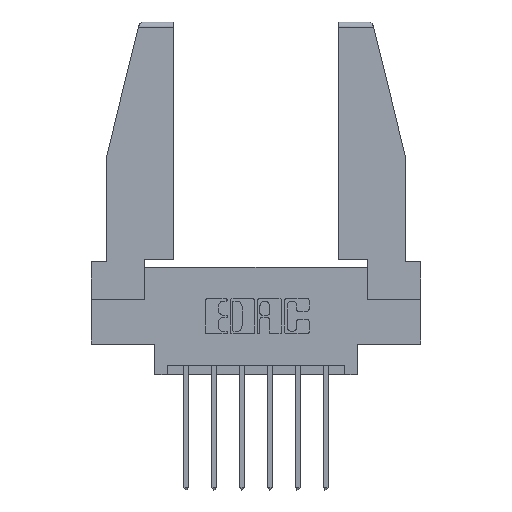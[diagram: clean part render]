
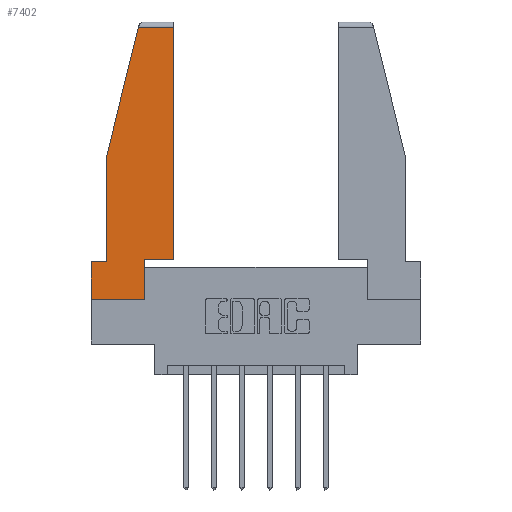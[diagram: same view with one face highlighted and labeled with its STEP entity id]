
A CAD part, top view. The second image highlights one B-rep face of the part: STEP entity #7402.
In plain terms, the highlighted planar face has unit normal (0, 0, 1).
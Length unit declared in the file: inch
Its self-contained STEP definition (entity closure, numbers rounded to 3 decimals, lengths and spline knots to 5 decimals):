
#170 = CARTESIAN_POINT ( 'NONE',  ( 0.297, 0.223, 0. ) ) ;
#223 = CARTESIAN_POINT ( 'NONE',  ( 0., 0.21, 0. ) ) ;
#345 = LINE ( 'NONE', #7909, #9709 ) ;
#404 = LINE ( 'NONE', #3564, #4568 ) ;
#1439 = EDGE_CURVE ( 'NONE', #1701, #2005, #3739, .T. ) ;
#1701 = VERTEX_POINT ( 'NONE', #3784 ) ;
#1802 = EDGE_CURVE ( 'NONE', #5195, #8325, #3585, .T. ) ;
#2005 = VERTEX_POINT ( 'NONE', #3179 ) ;
#2023 = DIRECTION ( 'NONE',  ( 1., 0., 0. ) ) ;
#2244 = CARTESIAN_POINT ( 'NONE',  ( 0., 0.21, 0. ) ) ;
#2677 = ORIENTED_EDGE ( 'NONE', *, *, #5609, .T. ) ;
#2774 = DIRECTION ( 'NONE',  ( 0., 1., 0. ) ) ;
#2810 = EDGE_CURVE ( 'NONE', #11155, #5195, #404, .T. ) ;
#3001 = ORIENTED_EDGE ( 'NONE', *, *, #6507, .T. ) ;
#3090 = ORIENTED_EDGE ( 'NONE', *, *, #7437, .T. ) ;
#3179 = CARTESIAN_POINT ( 'NONE',  ( 0.2636, 1.52, 0. ) ) ;
#3564 = CARTESIAN_POINT ( 'NONE',  ( 0.297, 0., 0. ) ) ;
#3585 = LINE ( 'NONE', #170, #5613 ) ;
#3739 = LINE ( 'NONE', #4511, #7657 ) ;
#3743 = DIRECTION ( 'NONE',  ( 1., 0., 0. ) ) ;
#3766 = CARTESIAN_POINT ( 'NONE',  ( 0., 0., 0. ) ) ;
#3771 = ORIENTED_EDGE ( 'NONE', *, *, #2810, .T. ) ;
#3784 = CARTESIAN_POINT ( 'NONE',  ( 0.461, 1.52, 0. ) ) ;
#4359 = EDGE_CURVE ( 'NONE', #9362, #11155, #7154, .T. ) ;
#4459 = CARTESIAN_POINT ( 'NONE',  ( 0.461, 0.223, 0. ) ) ;
#4460 = ORIENTED_EDGE ( 'NONE', *, *, #1802, .T. ) ;
#4511 = CARTESIAN_POINT ( 'NONE',  ( 0., 1.52, 0. ) ) ;
#4568 = VECTOR ( 'NONE', #5433, 39.37008 ) ;
#4641 = DIRECTION ( 'NONE',  ( -1., 0., 0. ) ) ;
#5174 = CARTESIAN_POINT ( 'NONE',  ( 0.297, 0.223, 0. ) ) ;
#5195 = VERTEX_POINT ( 'NONE', #5174 ) ;
#5255 = CARTESIAN_POINT ( 'NONE',  ( 0.297, 0., 0. ) ) ;
#5374 = DIRECTION ( 'NONE',  ( 0., -1., 0. ) ) ;
#5433 = DIRECTION ( 'NONE',  ( 0., 1., 0. ) ) ;
#5609 = EDGE_CURVE ( 'NONE', #8325, #1701, #7574, .T. ) ;
#5613 = VECTOR ( 'NONE', #3743, 39.37008 ) ;
#5628 = VERTEX_POINT ( 'NONE', #11048 ) ;
#5630 = CARTESIAN_POINT ( 'NONE',  ( 0., 0.21, 0. ) ) ;
#5664 = AXIS2_PLACEMENT_3D ( 'NONE', #3766, #7307, #10235 ) ;
#6057 = EDGE_CURVE ( 'NONE', #11297, #5628, #10888, .T. ) ;
#6272 = CARTESIAN_POINT ( 'NONE',  ( 0., 0., 0. ) ) ;
#6496 = VECTOR ( 'NONE', #8395, 39.37008 ) ;
#6507 = EDGE_CURVE ( 'NONE', #2005, #11297, #345, .T. ) ;
#6532 = VECTOR ( 'NONE', #5374, 39.37008 ) ;
#7154 = LINE ( 'NONE', #10879, #11902 ) ;
#7255 = VECTOR ( 'NONE', #2774, 39.37008 ) ;
#7307 = DIRECTION ( 'NONE',  ( 0., 0., 1. ) ) ;
#7402 = ADVANCED_FACE ( 'NONE', ( #8082 ), #11077, .T. ) ;
#7437 = EDGE_CURVE ( 'NONE', #5628, #10211, #10559, .T. ) ;
#7574 = LINE ( 'NONE', #8365, #7255 ) ;
#7657 = VECTOR ( 'NONE', #4641, 39.37008 ) ;
#7854 = EDGE_CURVE ( 'NONE', #10211, #9362, #8952, .T. ) ;
#7909 = CARTESIAN_POINT ( 'NONE',  ( 0.271, 1.55, 0. ) ) ;
#8082 = FACE_OUTER_BOUND ( 'NONE', #11638, .T. ) ;
#8325 = VERTEX_POINT ( 'NONE', #4459 ) ;
#8365 = CARTESIAN_POINT ( 'NONE',  ( 0.461, 0.223, 0. ) ) ;
#8394 = ORIENTED_EDGE ( 'NONE', *, *, #7854, .T. ) ;
#8395 = DIRECTION ( 'NONE',  ( -1., 0., 0. ) ) ;
#8705 = ORIENTED_EDGE ( 'NONE', *, *, #4359, .T. ) ;
#8952 = LINE ( 'NONE', #2244, #9105 ) ;
#9047 = CARTESIAN_POINT ( 'NONE',  ( 0.086, 0.8, 0. ) ) ;
#9105 = VECTOR ( 'NONE', #11491, 39.37008 ) ;
#9362 = VERTEX_POINT ( 'NONE', #6272 ) ;
#9465 = CARTESIAN_POINT ( 'NONE',  ( 0.086, 0.8, 0. ) ) ;
#9709 = VECTOR ( 'NONE', #11596, 39.37008 ) ;
#9996 = ORIENTED_EDGE ( 'NONE', *, *, #6057, .T. ) ;
#10211 = VERTEX_POINT ( 'NONE', #223 ) ;
#10235 = DIRECTION ( 'NONE',  ( 1., 0., 0. ) ) ;
#10559 = LINE ( 'NONE', #5630, #6496 ) ;
#10879 = CARTESIAN_POINT ( 'NONE',  ( 0., 0., 0. ) ) ;
#10888 = LINE ( 'NONE', #9047, #6532 ) ;
#11048 = CARTESIAN_POINT ( 'NONE',  ( 0.086, 0.21, 0. ) ) ;
#11077 = PLANE ( 'NONE',  #5664 ) ;
#11155 = VERTEX_POINT ( 'NONE', #5255 ) ;
#11297 = VERTEX_POINT ( 'NONE', #9465 ) ;
#11491 = DIRECTION ( 'NONE',  ( 0., -1., 0. ) ) ;
#11596 = DIRECTION ( 'NONE',  ( -0.239, -0.971, 0. ) ) ;
#11638 = EDGE_LOOP ( 'NONE', ( #2677, #11784, #3001, #9996, #3090, #8394, #8705, #3771, #4460 ) ) ;
#11784 = ORIENTED_EDGE ( 'NONE', *, *, #1439, .T. ) ;
#11902 = VECTOR ( 'NONE', #2023, 39.37008 ) ;
